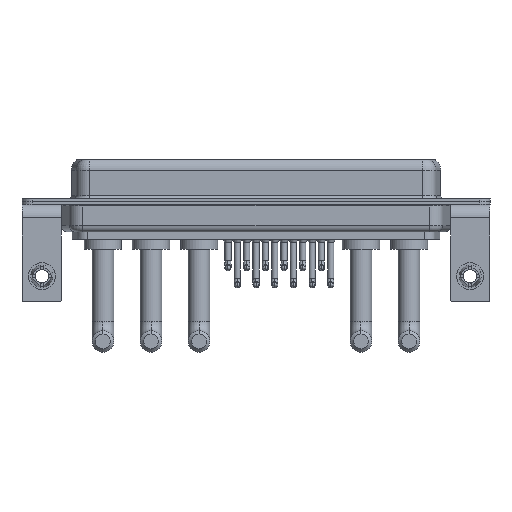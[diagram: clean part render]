
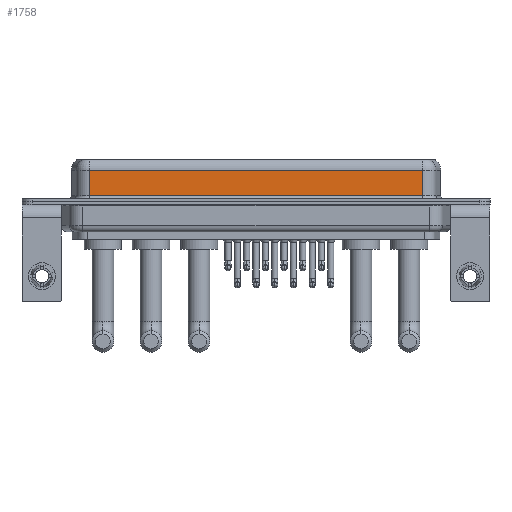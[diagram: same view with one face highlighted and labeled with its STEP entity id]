
A CAD part, front view. The second image highlights one B-rep face of the part: STEP entity #1758.
In plain terms, the highlighted planar face has unit normal (0, -1, 0).
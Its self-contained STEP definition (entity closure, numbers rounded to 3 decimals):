
#775 = LINE ( 'NONE', #7764, #6887 ) ;
#1758 = ADVANCED_FACE ( 'NONE', ( #18407 ), #22166, .F. ) ;
#2759 = LINE ( 'NONE', #13180, #19519 ) ;
#2788 = VERTEX_POINT ( 'NONE', #14660 ) ;
#2997 = LINE ( 'NONE', #21970, #5233 ) ;
#4486 = DIRECTION ( 'NONE',  ( 0., 0., -1. ) ) ;
#5233 = VECTOR ( 'NONE', #14682, 1000. ) ;
#6294 = AXIS2_PLACEMENT_3D ( 'NONE', #20115, #11454, #21823 ) ;
#6469 = DIRECTION ( 'NONE',  ( 1., 0., 0. ) ) ;
#6820 = VERTEX_POINT ( 'NONE', #13338 ) ;
#6887 = VECTOR ( 'NONE', #19748, 1000. ) ;
#7028 = CARTESIAN_POINT ( 'NONE',  ( 7.038, -3.95, 4.65 ) ) ;
#7764 = CARTESIAN_POINT ( 'NONE',  ( 56.462, -3.95, 4.65 ) ) ;
#10156 = VECTOR ( 'NONE', #6469, 1000. ) ;
#11094 = ORIENTED_EDGE ( 'NONE', *, *, #21029, .T. ) ;
#11454 = DIRECTION ( 'NONE',  ( 0., 1., 0. ) ) ;
#11809 = ORIENTED_EDGE ( 'NONE', *, *, #12346, .T. ) ;
#12346 = EDGE_CURVE ( 'NONE', #6820, #20975, #775, .T. ) ;
#12572 = VERTEX_POINT ( 'NONE', #16663 ) ;
#12985 = EDGE_CURVE ( 'NONE', #2788, #12572, #14599, .T. ) ;
#13180 = CARTESIAN_POINT ( 'NONE',  ( 7.038, -3.95, 6.4 ) ) ;
#13338 = CARTESIAN_POINT ( 'NONE',  ( 56.462, -3.95, 4.65 ) ) ;
#13814 = ORIENTED_EDGE ( 'NONE', *, *, #19812, .F. ) ;
#14599 = LINE ( 'NONE', #21550, #10156 ) ;
#14649 = ORIENTED_EDGE ( 'NONE', *, *, #12985, .T. ) ;
#14660 = CARTESIAN_POINT ( 'NONE',  ( 7.038, -3.95, 0.9 ) ) ;
#14682 = DIRECTION ( 'NONE',  ( 0., 0., -1. ) ) ;
#16663 = CARTESIAN_POINT ( 'NONE',  ( 56.462, -3.95, 0.9 ) ) ;
#18368 = EDGE_LOOP ( 'NONE', ( #13814, #11809, #11094, #14649 ) ) ;
#18407 = FACE_OUTER_BOUND ( 'NONE', #18368, .T. ) ;
#19519 = VECTOR ( 'NONE', #4486, 1000. ) ;
#19748 = DIRECTION ( 'NONE',  ( -1., 0., 0. ) ) ;
#19812 = EDGE_CURVE ( 'NONE', #6820, #12572, #2997, .T. ) ;
#20115 = CARTESIAN_POINT ( 'NONE',  ( 56.462, -3.95, 6.4 ) ) ;
#20975 = VERTEX_POINT ( 'NONE', #7028 ) ;
#21029 = EDGE_CURVE ( 'NONE', #20975, #2788, #2759, .T. ) ;
#21550 = CARTESIAN_POINT ( 'NONE',  ( 56.462, -3.95, 0.9 ) ) ;
#21823 = DIRECTION ( 'NONE',  ( 0., 0., 1. ) ) ;
#21970 = CARTESIAN_POINT ( 'NONE',  ( 56.462, -3.95, 6.4 ) ) ;
#22166 = PLANE ( 'NONE',  #6294 ) ;
